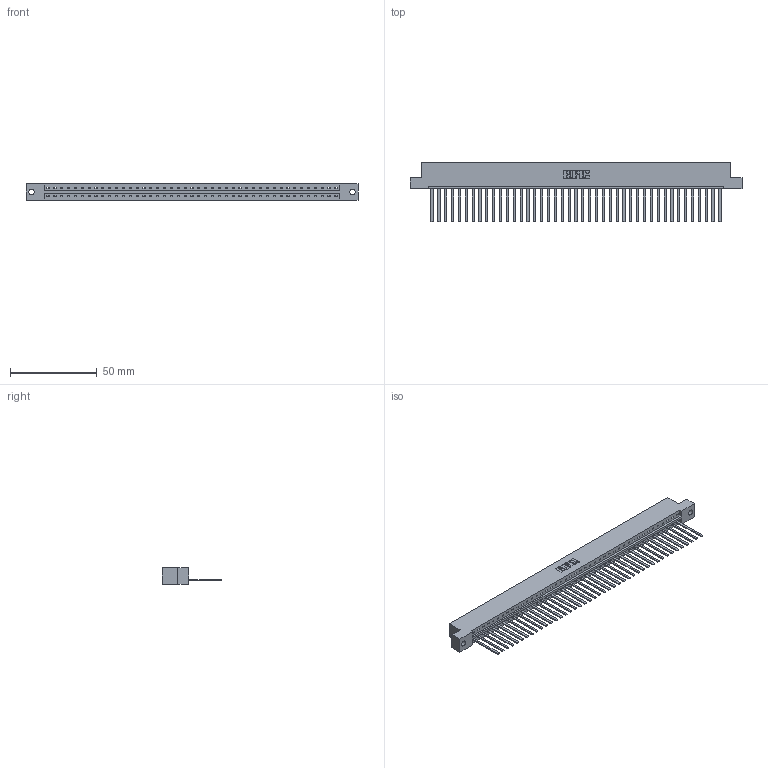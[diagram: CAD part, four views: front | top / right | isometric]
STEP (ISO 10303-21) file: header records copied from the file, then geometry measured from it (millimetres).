
FILE_DESCRIPTION (( 'STEP AP203' ), '1' );
FILE_NAME ('333-043-544-102.STEP', '2018-08-03T20:33:20', ( '' ), ( '' ), 'SwSTEP 2.0', 'SolidWorks 2016', '' );
FILE_SCHEMA (( 'CONFIG_CONTROL_DESIGN' ));
Length unit declared in the file: inch
Products named in the file (3): 333 Part_Flush - .128 Dia; 345-292-001_345-293-144; 333-043-544-102
Assembly tree (44 placements, depth 2):
  333-043-544-102
    333 Part_Flush - .128 Dia
    345-292-001_345-293-144  x43
Bounding box: 191.92 x 34.3 x 9.4 mm (x, y, z)
Volume: 19782.7 mm3; surface area: 22758.2 mm2
Topology: 44 solids, 44 shells, 2350 faces, 7105 edges, 4678 vertices
Faces by surface type: plane 1704, cylinder 646
Entity records: 25977 total; most frequent: CARTESIAN_POINT 4487, ORIENTED_EDGE 4466, DIRECTION 3779, EDGE_CURVE 2233, VECTOR 2109, LINE 2109, VERTEX_POINT 1486, AXIS2_PLACEMENT_3D 835
